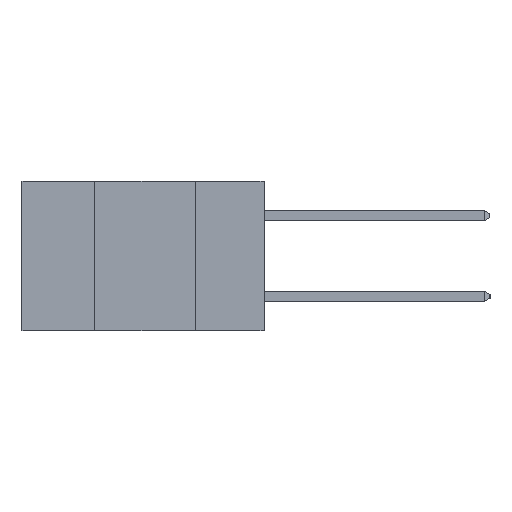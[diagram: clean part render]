
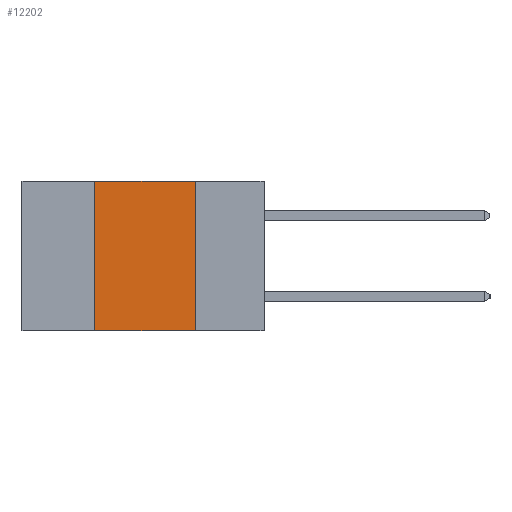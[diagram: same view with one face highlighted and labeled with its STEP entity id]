
A CAD part, left-side view. The second image highlights one B-rep face of the part: STEP entity #12202.
In plain terms, the highlighted planar face has unit normal (-1, 0, 0).
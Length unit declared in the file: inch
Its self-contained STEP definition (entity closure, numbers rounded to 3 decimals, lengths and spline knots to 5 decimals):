
#150 = LINE ( 'NONE', #12146, #11480 ) ;
#547 = VECTOR ( 'NONE', #12187, 39.37008 ) ;
#1273 = VERTEX_POINT ( 'NONE', #9026 ) ;
#1322 = VERTEX_POINT ( 'NONE', #11222 ) ;
#1632 = CARTESIAN_POINT ( 'NONE',  ( 0., 0.17, 0. ) ) ;
#1795 = VERTEX_POINT ( 'NONE', #10004 ) ;
#2507 = VERTEX_POINT ( 'NONE', #1632 ) ;
#2738 = ORIENTED_EDGE ( 'NONE', *, *, #13375, .T. ) ;
#2784 = DIRECTION ( 'NONE',  ( 0., 0., -1. ) ) ;
#2793 = DIRECTION ( 'NONE',  ( 1., 0., 0. ) ) ;
#2798 = PLANE ( 'NONE',  #13818 ) ;
#2940 = CARTESIAN_POINT ( 'NONE',  ( 0., 0.6, 0. ) ) ;
#3763 = LINE ( 'NONE', #12278, #547 ) ;
#3944 = VECTOR ( 'NONE', #14106, 39.37008 ) ;
#7835 = ORIENTED_EDGE ( 'NONE', *, *, #13205, .F. ) ;
#8166 = ORIENTED_EDGE ( 'NONE', *, *, #13346, .F. ) ;
#9026 = CARTESIAN_POINT ( 'NONE',  ( 0., 0.42, -0.37 ) ) ;
#9726 = LINE ( 'NONE', #13435, #13773 ) ;
#10004 = CARTESIAN_POINT ( 'NONE',  ( 0., 0.17, -0.37 ) ) ;
#11222 = CARTESIAN_POINT ( 'NONE',  ( 0., 0.42, 0. ) ) ;
#11480 = VECTOR ( 'NONE', #11506, 39.37008 ) ;
#11506 = DIRECTION ( 'NONE',  ( 0., -1., 0. ) ) ;
#11986 = LINE ( 'NONE', #13793, #3944 ) ;
#12146 = CARTESIAN_POINT ( 'NONE',  ( 0., 0.6, -0.37 ) ) ;
#12187 = DIRECTION ( 'NONE',  ( 0., 0., 1. ) ) ;
#12202 = ADVANCED_FACE ( 'NONE', ( #12211 ), #2798, .F. ) ;
#12211 = FACE_OUTER_BOUND ( 'NONE', #14098, .T. ) ;
#12278 = CARTESIAN_POINT ( 'NONE',  ( 0., 0.42, -0.37 ) ) ;
#13166 = EDGE_CURVE ( 'NONE', #2507, #1795, #11986, .T. ) ;
#13205 = EDGE_CURVE ( 'NONE', #1322, #2507, #9726, .T. ) ;
#13256 = DIRECTION ( 'NONE',  ( 0., -1., 0. ) ) ;
#13308 = ORIENTED_EDGE ( 'NONE', *, *, #13166, .F. ) ;
#13346 = EDGE_CURVE ( 'NONE', #1273, #1322, #3763, .T. ) ;
#13375 = EDGE_CURVE ( 'NONE', #1273, #1795, #150, .T. ) ;
#13435 = CARTESIAN_POINT ( 'NONE',  ( 0., 0.6, 0. ) ) ;
#13773 = VECTOR ( 'NONE', #13256, 39.37008 ) ;
#13793 = CARTESIAN_POINT ( 'NONE',  ( 0., 0.17, -0.37 ) ) ;
#13818 = AXIS2_PLACEMENT_3D ( 'NONE', #2940, #2793, #2784 ) ;
#14098 = EDGE_LOOP ( 'NONE', ( #13308, #7835, #8166, #2738 ) ) ;
#14106 = DIRECTION ( 'NONE',  ( 0., 0., -1. ) ) ;
